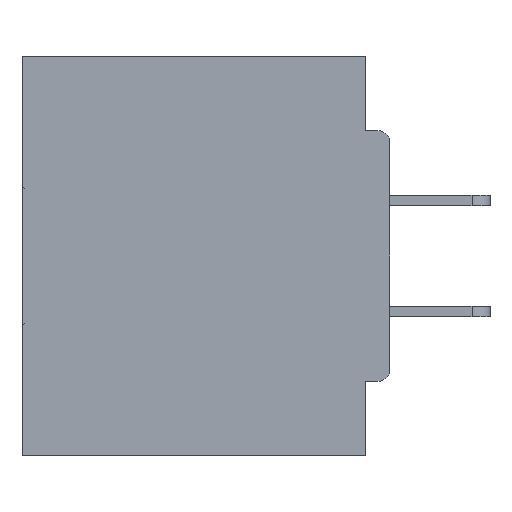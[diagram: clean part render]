
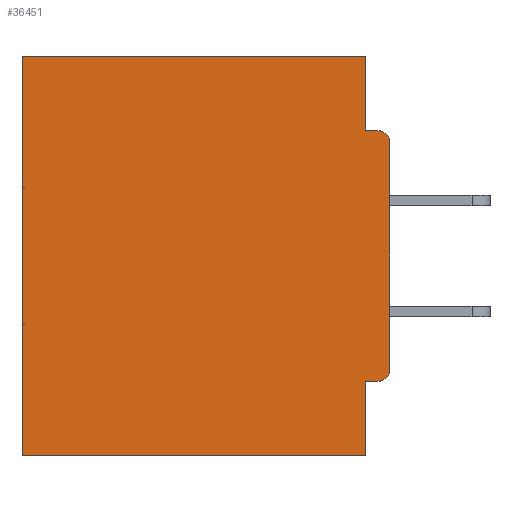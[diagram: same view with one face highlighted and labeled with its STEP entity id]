
A CAD part, left-side view. The second image highlights one B-rep face of the part: STEP entity #36451.
In plain terms, the highlighted planar face has unit normal (-1, 0, 0).
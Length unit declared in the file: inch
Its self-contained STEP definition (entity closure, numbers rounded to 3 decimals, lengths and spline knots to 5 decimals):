
#220 = CARTESIAN_POINT ( 'NONE',  ( 0.298, 0.46, 0. ) ) ;
#306 = DIRECTION ( 'NONE',  ( -1., 0., 0. ) ) ;
#354 = EDGE_LOOP ( 'NONE', ( #37848, #13713, #18446, #21211, #14095, #29961, #20218, #11669, #9633, #18095 ) ) ;
#2402 = VERTEX_POINT ( 'NONE', #23481 ) ;
#3109 = CARTESIAN_POINT ( 'NONE',  ( 0.298, 0.015, -0.1085 ) ) ;
#3314 = EDGE_CURVE ( 'NONE', #39113, #2402, #20681, .T. ) ;
#3387 = DIRECTION ( 'NONE',  ( 0., 0., -1. ) ) ;
#3635 = CARTESIAN_POINT ( 'NONE',  ( 0.298, 0., 0. ) ) ;
#4053 = CARTESIAN_POINT ( 'NONE',  ( 0.298, 0., -0.5 ) ) ;
#4205 = VECTOR ( 'NONE', #12449, 39.37008 ) ;
#5303 = CARTESIAN_POINT ( 'NONE',  ( 0.298, 0., -0.4065 ) ) ;
#5343 = DIRECTION ( 'NONE',  ( 0., 0., -1. ) ) ;
#5857 = CARTESIAN_POINT ( 'NONE',  ( 0.298, 0.031, -0.5 ) ) ;
#6341 = DIRECTION ( 'NONE',  ( 0., 1., 0. ) ) ;
#6437 = CARTESIAN_POINT ( 'NONE',  ( 0.298, 0.015, -0.0935 ) ) ;
#6461 = EDGE_CURVE ( 'NONE', #10220, #16132, #33580, .T. ) ;
#6775 = CARTESIAN_POINT ( 'NONE',  ( 0.298, 0.46, 0. ) ) ;
#7639 = DIRECTION ( 'NONE',  ( 0., 1., 0. ) ) ;
#7646 = CARTESIAN_POINT ( 'NONE',  ( 0.298, 0.015, -0.3915 ) ) ;
#7998 = VECTOR ( 'NONE', #7639, 39.37008 ) ;
#8442 = DIRECTION ( 'NONE',  ( 0., 1., 0. ) ) ;
#9633 = ORIENTED_EDGE ( 'NONE', *, *, #18706, .T. ) ;
#10022 = EDGE_CURVE ( 'NONE', #25384, #16132, #39892, .T. ) ;
#10220 = VERTEX_POINT ( 'NONE', #10923 ) ;
#10923 = CARTESIAN_POINT ( 'NONE',  ( 0.298, 0.031, -0.5 ) ) ;
#11669 = ORIENTED_EDGE ( 'NONE', *, *, #36965, .F. ) ;
#12442 = VERTEX_POINT ( 'NONE', #16148 ) ;
#12449 = DIRECTION ( 'NONE',  ( 0., 0., -1. ) ) ;
#13117 = LINE ( 'NONE', #22823, #34620 ) ;
#13679 = LINE ( 'NONE', #5303, #35148 ) ;
#13713 = ORIENTED_EDGE ( 'NONE', *, *, #18481, .F. ) ;
#14095 = ORIENTED_EDGE ( 'NONE', *, *, #10022, .T. ) ;
#14692 = DIRECTION ( 'NONE',  ( 0., -1., 0. ) ) ;
#15075 = CARTESIAN_POINT ( 'NONE',  ( 0.298, 0., 0. ) ) ;
#15184 = EDGE_CURVE ( 'NONE', #39848, #10220, #20613, .T. ) ;
#16132 = VERTEX_POINT ( 'NONE', #24829 ) ;
#16148 = CARTESIAN_POINT ( 'NONE',  ( 0.298, 0., -0.3915 ) ) ;
#16698 = CIRCLE ( 'NONE', #40910, 0.015 ) ;
#16762 = CARTESIAN_POINT ( 'NONE',  ( 0.298, 0.031, -0.5 ) ) ;
#17483 = CIRCLE ( 'NONE', #33692, 0.015 ) ;
#18095 = ORIENTED_EDGE ( 'NONE', *, *, #37244, .F. ) ;
#18225 = PLANE ( 'NONE',  #40064 ) ;
#18359 = DIRECTION ( 'NONE',  ( 1., 0., 0. ) ) ;
#18446 = ORIENTED_EDGE ( 'NONE', *, *, #3314, .F. ) ;
#18481 = EDGE_CURVE ( 'NONE', #2402, #33545, #32021, .T. ) ;
#18706 = EDGE_CURVE ( 'NONE', #38614, #12442, #16698, .T. ) ;
#20218 = ORIENTED_EDGE ( 'NONE', *, *, #15184, .F. ) ;
#20613 = LINE ( 'NONE', #5857, #4205 ) ;
#20681 = LINE ( 'NONE', #16762, #40507 ) ;
#21211 = ORIENTED_EDGE ( 'NONE', *, *, #30996, .T. ) ;
#22147 = LINE ( 'NONE', #3635, #31280 ) ;
#22823 = CARTESIAN_POINT ( 'NONE',  ( 0.298, 0., 0. ) ) ;
#23346 = CARTESIAN_POINT ( 'NONE',  ( 0.298, 0.031, -0.4065 ) ) ;
#23481 = CARTESIAN_POINT ( 'NONE',  ( 0.298, 0.031, -0.0935 ) ) ;
#24300 = VERTEX_POINT ( 'NONE', #40940 ) ;
#24829 = CARTESIAN_POINT ( 'NONE',  ( 0.298, 0.46, -0.5 ) ) ;
#25384 = VERTEX_POINT ( 'NONE', #220 ) ;
#25557 = CARTESIAN_POINT ( 'NONE',  ( 0.298, 0.031, 0. ) ) ;
#25992 = DIRECTION ( 'NONE',  ( 0., 0., -1. ) ) ;
#26081 = DIRECTION ( 'NONE',  ( 0., 0., -1. ) ) ;
#29961 = ORIENTED_EDGE ( 'NONE', *, *, #6461, .F. ) ;
#30996 = EDGE_CURVE ( 'NONE', #39113, #25384, #22147, .T. ) ;
#31280 = VECTOR ( 'NONE', #6341, 39.37008 ) ;
#31408 = EDGE_CURVE ( 'NONE', #24300, #33545, #17483, .T. ) ;
#31495 = VECTOR ( 'NONE', #14692, 39.37008 ) ;
#32021 = LINE ( 'NONE', #40336, #31495 ) ;
#33287 = FACE_OUTER_BOUND ( 'NONE', #354, .T. ) ;
#33306 = VECTOR ( 'NONE', #39305, 39.37008 ) ;
#33545 = VERTEX_POINT ( 'NONE', #6437 ) ;
#33580 = LINE ( 'NONE', #4053, #7998 ) ;
#33692 = AXIS2_PLACEMENT_3D ( 'NONE', #3109, #306, #26081 ) ;
#34620 = VECTOR ( 'NONE', #3387, 39.37008 ) ;
#35148 = VECTOR ( 'NONE', #8442, 39.37008 ) ;
#36451 = ADVANCED_FACE ( 'NONE', ( #33287 ), #18225, .F. ) ;
#36911 = DIRECTION ( 'NONE',  ( 0., 0., -1. ) ) ;
#36965 = EDGE_CURVE ( 'NONE', #38614, #39848, #13679, .T. ) ;
#37244 = EDGE_CURVE ( 'NONE', #24300, #12442, #13117, .T. ) ;
#37848 = ORIENTED_EDGE ( 'NONE', *, *, #31408, .T. ) ;
#38614 = VERTEX_POINT ( 'NONE', #41963 ) ;
#39113 = VERTEX_POINT ( 'NONE', #25557 ) ;
#39305 = DIRECTION ( 'NONE',  ( 0., 0., -1. ) ) ;
#39848 = VERTEX_POINT ( 'NONE', #23346 ) ;
#39892 = LINE ( 'NONE', #6775, #33306 ) ;
#40064 = AXIS2_PLACEMENT_3D ( 'NONE', #15075, #18359, #5343 ) ;
#40292 = DIRECTION ( 'NONE',  ( -1., 0., 0. ) ) ;
#40336 = CARTESIAN_POINT ( 'NONE',  ( 0.298, 0., -0.0935 ) ) ;
#40507 = VECTOR ( 'NONE', #25992, 39.37008 ) ;
#40910 = AXIS2_PLACEMENT_3D ( 'NONE', #7646, #40292, #36911 ) ;
#40940 = CARTESIAN_POINT ( 'NONE',  ( 0.298, 0., -0.1085 ) ) ;
#41963 = CARTESIAN_POINT ( 'NONE',  ( 0.298, 0.015, -0.4065 ) ) ;
